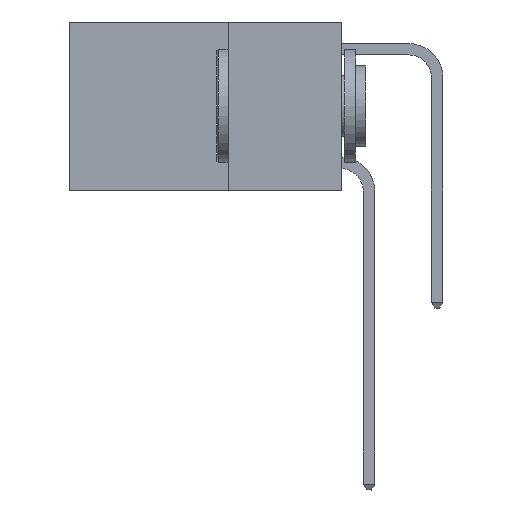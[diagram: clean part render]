
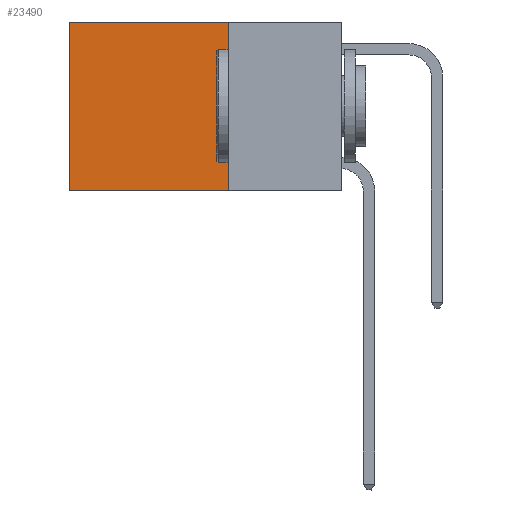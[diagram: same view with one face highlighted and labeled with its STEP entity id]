
A CAD part, left-side view. The second image highlights one B-rep face of the part: STEP entity #23490.
In plain terms, the highlighted planar face has unit normal (-1, 0, 0).
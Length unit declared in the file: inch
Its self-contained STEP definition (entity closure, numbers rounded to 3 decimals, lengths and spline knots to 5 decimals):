
#1239 = LINE ( 'NONE', #10113, #5470 ) ;
#1375 = LINE ( 'NONE', #15071, #20064 ) ;
#1382 = LINE ( 'NONE', #7649, #7552 ) ;
#1891 = VECTOR ( 'NONE', #2310, 39.37008 ) ;
#2310 = DIRECTION ( 'NONE',  ( 0., 1., 0. ) ) ;
#2543 = DIRECTION ( 'NONE',  ( 1., 0., 0. ) ) ;
#2653 = VERTEX_POINT ( 'NONE', #3541 ) ;
#2723 = EDGE_LOOP ( 'NONE', ( #27831, #18172, #15120, #6283 ) ) ;
#2811 = CARTESIAN_POINT ( 'NONE',  ( 0.2625, 0.25, 0. ) ) ;
#3541 = CARTESIAN_POINT ( 'NONE',  ( 0.2625, 0.6, 0. ) ) ;
#4459 = CARTESIAN_POINT ( 'NONE',  ( 0.2625, 0.25, 0. ) ) ;
#4611 = AXIS2_PLACEMENT_3D ( 'NONE', #2811, #2543, #17969 ) ;
#5292 = FACE_OUTER_BOUND ( 'NONE', #2723, .T. ) ;
#5470 = VECTOR ( 'NONE', #23635, 39.37008 ) ;
#5899 = DIRECTION ( 'NONE',  ( 0., 1., 0. ) ) ;
#6283 = ORIENTED_EDGE ( 'NONE', *, *, #15594, .T. ) ;
#7552 = VECTOR ( 'NONE', #5899, 39.37008 ) ;
#7649 = CARTESIAN_POINT ( 'NONE',  ( 0.2625, 0.25, 0. ) ) ;
#8408 = VERTEX_POINT ( 'NONE', #4459 ) ;
#10113 = CARTESIAN_POINT ( 'NONE',  ( 0.2625, 0.6, 0. ) ) ;
#13232 = CARTESIAN_POINT ( 'NONE',  ( 0.2625, 0.25, -0.37 ) ) ;
#13380 = VERTEX_POINT ( 'NONE', #13232 ) ;
#14188 = CARTESIAN_POINT ( 'NONE',  ( 0.2625, 0.6, -0.37 ) ) ;
#15071 = CARTESIAN_POINT ( 'NONE',  ( 0.2625, 0.25, 0. ) ) ;
#15120 = ORIENTED_EDGE ( 'NONE', *, *, #28707, .F. ) ;
#15594 = EDGE_CURVE ( 'NONE', #8408, #2653, #1382, .T. ) ;
#16081 = PLANE ( 'NONE',  #4611 ) ;
#17969 = DIRECTION ( 'NONE',  ( 0., 0., -1. ) ) ;
#18154 = CARTESIAN_POINT ( 'NONE',  ( 0.2625, 0.25, -0.37 ) ) ;
#18172 = ORIENTED_EDGE ( 'NONE', *, *, #26574, .F. ) ;
#19273 = VERTEX_POINT ( 'NONE', #14188 ) ;
#20064 = VECTOR ( 'NONE', #21464, 39.37008 ) ;
#21464 = DIRECTION ( 'NONE',  ( 0., 0., -1. ) ) ;
#21815 = EDGE_CURVE ( 'NONE', #2653, #19273, #1239, .T. ) ;
#22118 = LINE ( 'NONE', #18154, #1891 ) ;
#23490 = ADVANCED_FACE ( 'NONE', ( #5292 ), #16081, .F. ) ;
#23635 = DIRECTION ( 'NONE',  ( 0., 0., -1. ) ) ;
#26574 = EDGE_CURVE ( 'NONE', #13380, #19273, #22118, .T. ) ;
#27831 = ORIENTED_EDGE ( 'NONE', *, *, #21815, .T. ) ;
#28707 = EDGE_CURVE ( 'NONE', #8408, #13380, #1375, .T. ) ;
